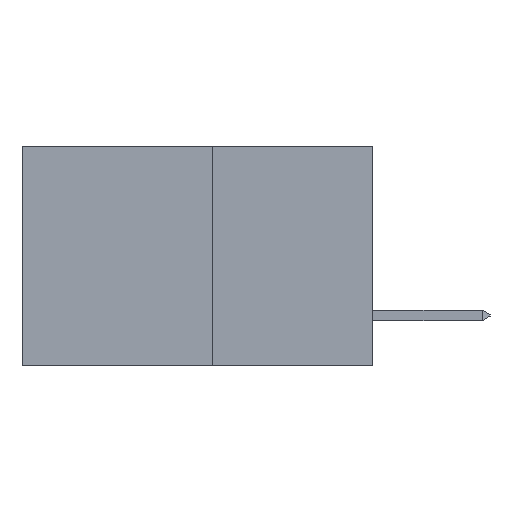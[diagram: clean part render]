
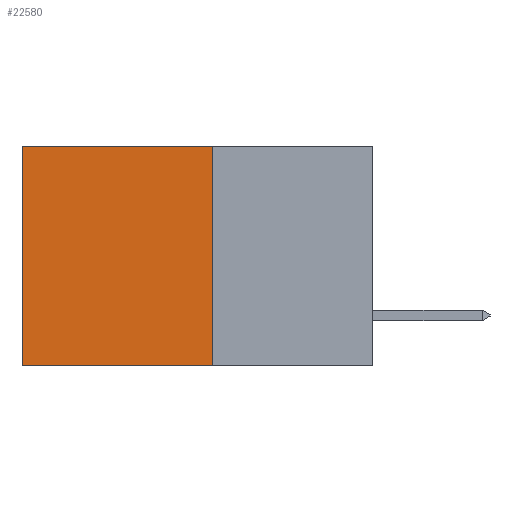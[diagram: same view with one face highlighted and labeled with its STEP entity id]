
A CAD part, left-side view. The second image highlights one B-rep face of the part: STEP entity #22580.
In plain terms, the highlighted planar face has unit normal (-1, 0, 0).
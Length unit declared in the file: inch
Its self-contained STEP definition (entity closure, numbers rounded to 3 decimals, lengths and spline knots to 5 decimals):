
#1033 = CARTESIAN_POINT ( 'NONE',  ( 0.277, 0.27, -0.37 ) ) ;
#1714 = LINE ( 'NONE', #9424, #12119 ) ;
#2503 = ORIENTED_EDGE ( 'NONE', *, *, #12582, .T. ) ;
#3556 = VERTEX_POINT ( 'NONE', #11150 ) ;
#3892 = DIRECTION ( 'NONE',  ( 0., 1., 0. ) ) ;
#4623 = DIRECTION ( 'NONE',  ( 1., 0., 0. ) ) ;
#5748 = CARTESIAN_POINT ( 'NONE',  ( 0.277, 0.59, 0. ) ) ;
#6004 = ORIENTED_EDGE ( 'NONE', *, *, #12905, .T. ) ;
#6005 = VERTEX_POINT ( 'NONE', #5748 ) ;
#7404 = EDGE_CURVE ( 'NONE', #27312, #18485, #23516, .T. ) ;
#7640 = ORIENTED_EDGE ( 'NONE', *, *, #19020, .F. ) ;
#9424 = CARTESIAN_POINT ( 'NONE',  ( 0.277, 0.59, -0.37 ) ) ;
#10773 = VECTOR ( 'NONE', #3892, 39.37008 ) ;
#11150 = CARTESIAN_POINT ( 'NONE',  ( 0.277, 0.59, -0.37 ) ) ;
#12119 = VECTOR ( 'NONE', #22801, 39.37008 ) ;
#12582 = EDGE_CURVE ( 'NONE', #27312, #6005, #21246, .T. ) ;
#12905 = EDGE_CURVE ( 'NONE', #6005, #3556, #1714, .T. ) ;
#13452 = PLANE ( 'NONE',  #14003 ) ;
#14003 = AXIS2_PLACEMENT_3D ( 'NONE', #17936, #4623, #20229 ) ;
#14309 = DIRECTION ( 'NONE',  ( 0., 1., 0. ) ) ;
#15057 = ORIENTED_EDGE ( 'NONE', *, *, #7404, .F. ) ;
#15995 = LINE ( 'NONE', #1033, #27144 ) ;
#16245 = CARTESIAN_POINT ( 'NONE',  ( 0.277, 0.27, -0.37 ) ) ;
#17936 = CARTESIAN_POINT ( 'NONE',  ( 0.277, 0.27, -0.37 ) ) ;
#18485 = VERTEX_POINT ( 'NONE', #21908 ) ;
#19020 = EDGE_CURVE ( 'NONE', #18485, #3556, #15995, .T. ) ;
#20229 = DIRECTION ( 'NONE',  ( 0., 0., -1. ) ) ;
#21246 = LINE ( 'NONE', #23879, #10773 ) ;
#21908 = CARTESIAN_POINT ( 'NONE',  ( 0.277, 0.27, -0.37 ) ) ;
#21960 = EDGE_LOOP ( 'NONE', ( #6004, #7640, #15057, #2503 ) ) ;
#22580 = ADVANCED_FACE ( 'NONE', ( #26747 ), #13452, .F. ) ;
#22801 = DIRECTION ( 'NONE',  ( 0., 0., -1. ) ) ;
#22830 = VECTOR ( 'NONE', #25241, 39.37008 ) ;
#23516 = LINE ( 'NONE', #16245, #22830 ) ;
#23879 = CARTESIAN_POINT ( 'NONE',  ( 0.277, 0.27, 0. ) ) ;
#25241 = DIRECTION ( 'NONE',  ( 0., 0., -1. ) ) ;
#26747 = FACE_OUTER_BOUND ( 'NONE', #21960, .T. ) ;
#27016 = CARTESIAN_POINT ( 'NONE',  ( 0.277, 0.27, 0. ) ) ;
#27144 = VECTOR ( 'NONE', #14309, 39.37008 ) ;
#27312 = VERTEX_POINT ( 'NONE', #27016 ) ;
